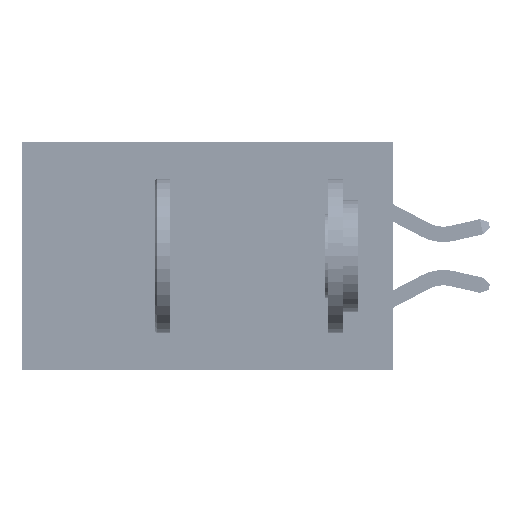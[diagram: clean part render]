
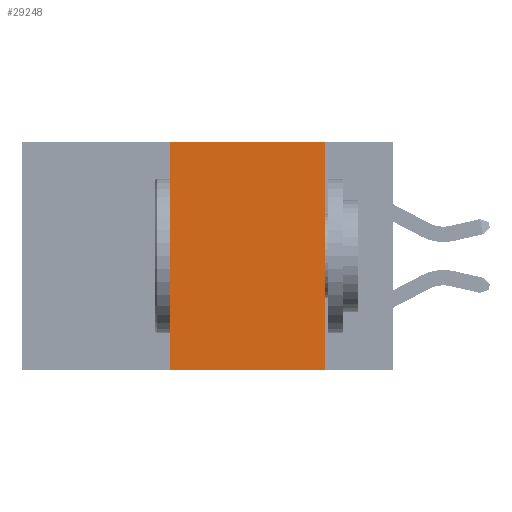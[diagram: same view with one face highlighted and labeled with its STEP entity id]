
A CAD part, left-side view. The second image highlights one B-rep face of the part: STEP entity #29248.
In plain terms, the highlighted planar face has unit normal (-1, 0, 0).
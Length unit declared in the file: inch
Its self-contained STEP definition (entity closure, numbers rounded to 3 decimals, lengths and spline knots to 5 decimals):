
#824 = LINE ( 'NONE', #7904, #35521 ) ;
#4066 = VERTEX_POINT ( 'NONE', #28489 ) ;
#4682 = VERTEX_POINT ( 'NONE', #11789 ) ;
#4894 = EDGE_LOOP ( 'NONE', ( #10635, #47815, #10725, #28101 ) ) ;
#5012 = AXIS2_PLACEMENT_3D ( 'NONE', #22390, #5660, #25771 ) ;
#5660 = DIRECTION ( 'NONE',  ( 1., 0., 0. ) ) ;
#6015 = VECTOR ( 'NONE', #31965, 39.37008 ) ;
#6502 = VECTOR ( 'NONE', #15049, 39.37008 ) ;
#7904 = CARTESIAN_POINT ( 'NONE',  ( 0., 0.11, 0. ) ) ;
#9784 = LINE ( 'NONE', #20196, #6015 ) ;
#10635 = ORIENTED_EDGE ( 'NONE', *, *, #20406, .F. ) ;
#10725 = ORIENTED_EDGE ( 'NONE', *, *, #28310, .F. ) ;
#11677 = CARTESIAN_POINT ( 'NONE',  ( 0., 0.36, 0. ) ) ;
#11789 = CARTESIAN_POINT ( 'NONE',  ( 0., 0.36, 0. ) ) ;
#14875 = VERTEX_POINT ( 'NONE', #36797 ) ;
#15049 = DIRECTION ( 'NONE',  ( 0., 0., 1. ) ) ;
#16315 = EDGE_CURVE ( 'NONE', #14875, #4066, #31408, .T. ) ;
#16612 = CARTESIAN_POINT ( 'NONE',  ( 0., 0.11, 0. ) ) ;
#17439 = CARTESIAN_POINT ( 'NONE',  ( 0., 0.6, -0.37 ) ) ;
#17680 = EDGE_CURVE ( 'NONE', #4682, #47332, #9784, .T. ) ;
#17794 = DIRECTION ( 'NONE',  ( 0., -1., 0. ) ) ;
#20196 = CARTESIAN_POINT ( 'NONE',  ( 0., 0.6, 0. ) ) ;
#20406 = EDGE_CURVE ( 'NONE', #47332, #4066, #824, .T. ) ;
#21530 = FACE_OUTER_BOUND ( 'NONE', #4894, .T. ) ;
#22390 = CARTESIAN_POINT ( 'NONE',  ( 0., 0.6, 0. ) ) ;
#22867 = LINE ( 'NONE', #11677, #6502 ) ;
#25771 = DIRECTION ( 'NONE',  ( 0., 0., -1. ) ) ;
#28101 = ORIENTED_EDGE ( 'NONE', *, *, #16315, .T. ) ;
#28310 = EDGE_CURVE ( 'NONE', #14875, #4682, #22867, .T. ) ;
#28489 = CARTESIAN_POINT ( 'NONE',  ( 0., 0.11, -0.37 ) ) ;
#29248 = ADVANCED_FACE ( 'NONE', ( #21530 ), #50067, .F. ) ;
#31408 = LINE ( 'NONE', #17439, #44631 ) ;
#31965 = DIRECTION ( 'NONE',  ( 0., -1., 0. ) ) ;
#35521 = VECTOR ( 'NONE', #51950, 39.37008 ) ;
#36797 = CARTESIAN_POINT ( 'NONE',  ( 0., 0.36, -0.37 ) ) ;
#44631 = VECTOR ( 'NONE', #17794, 39.37008 ) ;
#47332 = VERTEX_POINT ( 'NONE', #16612 ) ;
#47815 = ORIENTED_EDGE ( 'NONE', *, *, #17680, .F. ) ;
#50067 = PLANE ( 'NONE',  #5012 ) ;
#51950 = DIRECTION ( 'NONE',  ( 0., 0., -1. ) ) ;
